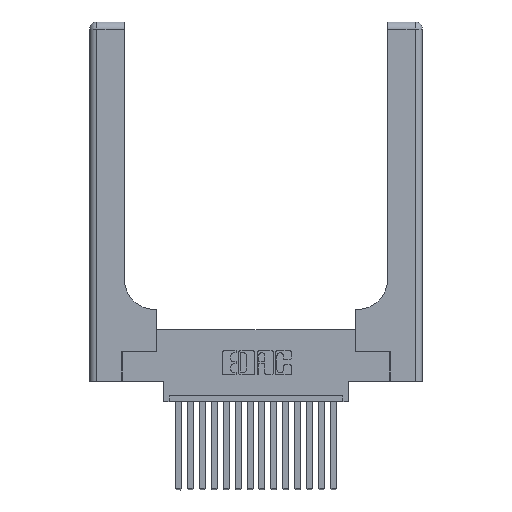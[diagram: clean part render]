
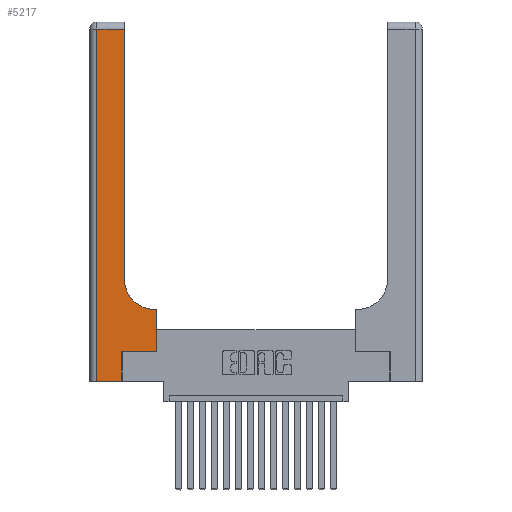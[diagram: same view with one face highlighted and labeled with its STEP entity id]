
A CAD part, top view. The second image highlights one B-rep face of the part: STEP entity #5217.
In plain terms, the highlighted planar face has unit normal (0, 0, 1).
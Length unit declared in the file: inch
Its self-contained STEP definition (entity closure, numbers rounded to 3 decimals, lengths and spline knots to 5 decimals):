
#472 = CARTESIAN_POINT ( 'NONE',  ( 0.5585, 0.25, 0.37 ) ) ;
#790 = VECTOR ( 'NONE', #1459, 39.37008 ) ;
#969 = VERTEX_POINT ( 'NONE', #17091 ) ;
#1070 = CARTESIAN_POINT ( 'NONE',  ( 0.269, 0.25, 0.37 ) ) ;
#1440 = ORIENTED_EDGE ( 'NONE', *, *, #12525, .T. ) ;
#1459 = DIRECTION ( 'NONE',  ( 0., 1., 0. ) ) ;
#2013 = ORIENTED_EDGE ( 'NONE', *, *, #18288, .T. ) ;
#2215 = CARTESIAN_POINT ( 'NONE',  ( 0., 3., 0.37 ) ) ;
#2961 = VECTOR ( 'NONE', #10426, 39.37008 ) ;
#2986 = LINE ( 'NONE', #15958, #16578 ) ;
#3054 = EDGE_CURVE ( 'NONE', #16017, #12238, #13230, .T. ) ;
#3619 = DIRECTION ( 'NONE',  ( 0., 1., 0. ) ) ;
#3841 = VERTEX_POINT ( 'NONE', #10320 ) ;
#3918 = LINE ( 'NONE', #5003, #15134 ) ;
#4418 = EDGE_CURVE ( 'NONE', #12238, #4927, #12708, .T. ) ;
#4482 = DIRECTION ( 'NONE',  ( 1., 0., 0. ) ) ;
#4687 = CARTESIAN_POINT ( 'NONE',  ( 0.5585, 0.6, 0.37 ) ) ;
#4743 = ORIENTED_EDGE ( 'NONE', *, *, #19136, .T. ) ;
#4927 = VERTEX_POINT ( 'NONE', #11188 ) ;
#5003 = CARTESIAN_POINT ( 'NONE',  ( 0.06, 3., 0.37 ) ) ;
#5100 = LINE ( 'NONE', #14493, #8595 ) ;
#5217 = ADVANCED_FACE ( 'NONE', ( #12690 ), #14231, .F. ) ;
#5302 = VECTOR ( 'NONE', #5604, 39.37008 ) ;
#5318 = DIRECTION ( 'NONE',  ( -1., 0., 0. ) ) ;
#5468 = CARTESIAN_POINT ( 'NONE',  ( 0.06, 0., 0.37 ) ) ;
#5604 = DIRECTION ( 'NONE',  ( 1., 0., 0. ) ) ;
#7215 = LINE ( 'NONE', #472, #9565 ) ;
#7297 = CARTESIAN_POINT ( 'NONE',  ( 0.5415, 0.85, 0.37 ) ) ;
#7452 = CARTESIAN_POINT ( 'NONE',  ( 0., 0., 0.37 ) ) ;
#7461 = AXIS2_PLACEMENT_3D ( 'NONE', #2215, #17176, #18818 ) ;
#7508 = DIRECTION ( 'NONE',  ( 0., 0., -1. ) ) ;
#7715 = CARTESIAN_POINT ( 'NONE',  ( 0.2915, 3., 0.37 ) ) ;
#7906 = LINE ( 'NONE', #7452, #2961 ) ;
#8282 = ORIENTED_EDGE ( 'NONE', *, *, #18417, .T. ) ;
#8382 = VERTEX_POINT ( 'NONE', #12115 ) ;
#8595 = VECTOR ( 'NONE', #14240, 39.37008 ) ;
#9565 = VECTOR ( 'NONE', #3619, 39.37008 ) ;
#10169 = LINE ( 'NONE', #7715, #790 ) ;
#10320 = CARTESIAN_POINT ( 'NONE',  ( 0.269, 0.25, 0.37 ) ) ;
#10426 = DIRECTION ( 'NONE',  ( 1., 0., 0. ) ) ;
#10449 = ORIENTED_EDGE ( 'NONE', *, *, #18551, .T. ) ;
#10919 = VECTOR ( 'NONE', #15891, 39.37008 ) ;
#11188 = CARTESIAN_POINT ( 'NONE',  ( 0.2915, 0.85, 0.37 ) ) ;
#11936 = EDGE_CURVE ( 'NONE', #17324, #19441, #7906, .T. ) ;
#12115 = CARTESIAN_POINT ( 'NONE',  ( 0.06, 2.94, 0.37 ) ) ;
#12238 = VERTEX_POINT ( 'NONE', #17492 ) ;
#12525 = EDGE_CURVE ( 'NONE', #4927, #16483, #10169, .T. ) ;
#12690 = FACE_OUTER_BOUND ( 'NONE', #14085, .T. ) ;
#12708 = CIRCLE ( 'NONE', #16870, 0.25 ) ;
#13230 = LINE ( 'NONE', #14484, #10919 ) ;
#14085 = EDGE_LOOP ( 'NONE', ( #1440, #10449, #8282, #16047, #17864, #4743, #2013, #18651, #16511 ) ) ;
#14106 = DIRECTION ( 'NONE',  ( 0., -1., 0. ) ) ;
#14231 = PLANE ( 'NONE',  #7461 ) ;
#14240 = DIRECTION ( 'NONE',  ( 0., 1., 0. ) ) ;
#14484 = CARTESIAN_POINT ( 'NONE',  ( 0.2915, 0.6, 0.37 ) ) ;
#14493 = CARTESIAN_POINT ( 'NONE',  ( 0.269, 0., 0.37 ) ) ;
#14821 = CARTESIAN_POINT ( 'NONE',  ( 0.2915, 2.94, 0.37 ) ) ;
#15134 = VECTOR ( 'NONE', #14106, 39.37008 ) ;
#15891 = DIRECTION ( 'NONE',  ( -1., 0., 0. ) ) ;
#15958 = CARTESIAN_POINT ( 'NONE',  ( 0., 2.94, 0.37 ) ) ;
#16017 = VERTEX_POINT ( 'NONE', #4687 ) ;
#16047 = ORIENTED_EDGE ( 'NONE', *, *, #11936, .T. ) ;
#16483 = VERTEX_POINT ( 'NONE', #14821 ) ;
#16511 = ORIENTED_EDGE ( 'NONE', *, *, #4418, .T. ) ;
#16578 = VECTOR ( 'NONE', #5318, 39.37008 ) ;
#16676 = CARTESIAN_POINT ( 'NONE',  ( 0.269, 0., 0.37 ) ) ;
#16870 = AXIS2_PLACEMENT_3D ( 'NONE', #7297, #7508, #4482 ) ;
#17091 = CARTESIAN_POINT ( 'NONE',  ( 0.5585, 0.25, 0.37 ) ) ;
#17176 = DIRECTION ( 'NONE',  ( 0., 0., -1. ) ) ;
#17324 = VERTEX_POINT ( 'NONE', #5468 ) ;
#17492 = CARTESIAN_POINT ( 'NONE',  ( 0.5415, 0.6, 0.37 ) ) ;
#17721 = LINE ( 'NONE', #1070, #5302 ) ;
#17864 = ORIENTED_EDGE ( 'NONE', *, *, #18539, .T. ) ;
#18288 = EDGE_CURVE ( 'NONE', #969, #16017, #7215, .T. ) ;
#18417 = EDGE_CURVE ( 'NONE', #8382, #17324, #3918, .T. ) ;
#18539 = EDGE_CURVE ( 'NONE', #19441, #3841, #5100, .T. ) ;
#18551 = EDGE_CURVE ( 'NONE', #16483, #8382, #2986, .T. ) ;
#18651 = ORIENTED_EDGE ( 'NONE', *, *, #3054, .T. ) ;
#18818 = DIRECTION ( 'NONE',  ( -1., 0., 0. ) ) ;
#19136 = EDGE_CURVE ( 'NONE', #3841, #969, #17721, .T. ) ;
#19441 = VERTEX_POINT ( 'NONE', #16676 ) ;
